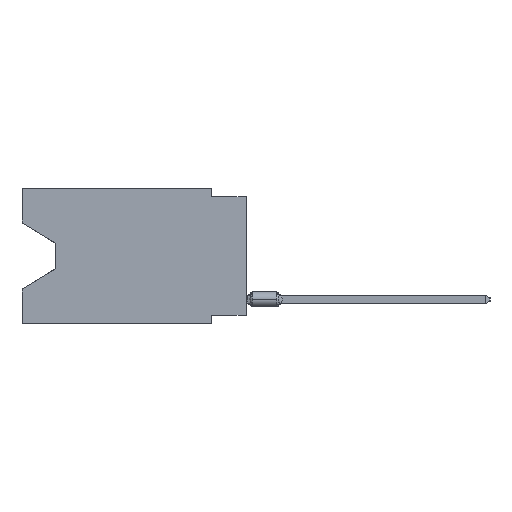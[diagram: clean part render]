
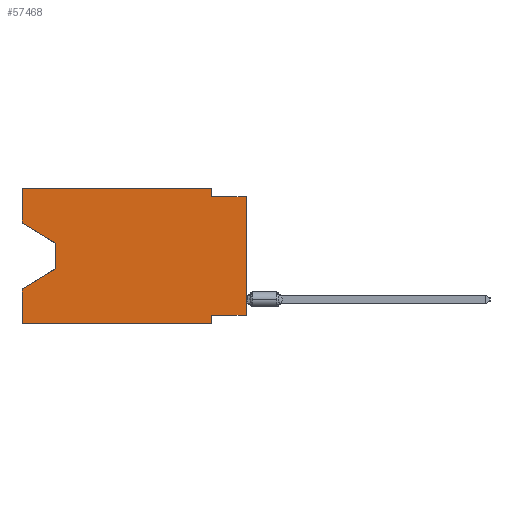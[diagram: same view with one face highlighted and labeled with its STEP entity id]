
A CAD part, left-side view. The second image highlights one B-rep face of the part: STEP entity #57468.
In plain terms, the highlighted planar face has unit normal (-1, 0, 0).
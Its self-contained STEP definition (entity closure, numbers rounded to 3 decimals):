
#312 = VERTEX_POINT ( 'NONE', #64722 ) ;
#390 = VERTEX_POINT ( 'NONE', #60776 ) ;
#616 = LINE ( 'NONE', #49810, #27023 ) ;
#1805 = VECTOR ( 'NONE', #11843, 1000. ) ;
#2131 = CARTESIAN_POINT ( 'NONE',  ( 0., 2.54, 0. ) ) ;
#2277 = DIRECTION ( 'NONE',  ( 0., 0., 1. ) ) ;
#3810 = VERTEX_POINT ( 'NONE', #54283 ) ;
#4911 = DIRECTION ( 'NONE',  ( 0., 0., -1. ) ) ;
#5344 = ORIENTED_EDGE ( 'NONE', *, *, #46273, .F. ) ;
#6207 = LINE ( 'NONE', #26187, #10376 ) ;
#6479 = EDGE_CURVE ( 'NONE', #29815, #59189, #6207, .T. ) ;
#7661 = VECTOR ( 'NONE', #58442, 1000. ) ;
#8578 = ORIENTED_EDGE ( 'NONE', *, *, #23154, .F. ) ;
#8912 = VERTEX_POINT ( 'NONE', #18530 ) ;
#9958 = VECTOR ( 'NONE', #48693, 1000. ) ;
#10316 = ORIENTED_EDGE ( 'NONE', *, *, #39422, .F. ) ;
#10376 = VECTOR ( 'NONE', #10479, 1000. ) ;
#10479 = DIRECTION ( 'NONE',  ( 0., 0., 1. ) ) ;
#11692 = CARTESIAN_POINT ( 'NONE',  ( 0., 16.383, 0. ) ) ;
#11843 = DIRECTION ( 'NONE',  ( 0., -1., 0. ) ) ;
#12703 = CARTESIAN_POINT ( 'NONE',  ( 0., 16.383, 0. ) ) ;
#13539 = ORIENTED_EDGE ( 'NONE', *, *, #14129, .T. ) ;
#14129 = EDGE_CURVE ( 'NONE', #24003, #54832, #16486, .T. ) ;
#15147 = VECTOR ( 'NONE', #36463, 1000. ) ;
#15238 = LINE ( 'NONE', #35218, #9958 ) ;
#15255 = CARTESIAN_POINT ( 'NONE',  ( 0., 0., -9.271 ) ) ;
#15559 = CARTESIAN_POINT ( 'NONE',  ( 0., 13.97, -4.013 ) ) ;
#15710 = EDGE_CURVE ( 'NONE', #23939, #8912, #48257, .T. ) ;
#16486 = LINE ( 'NONE', #56502, #15147 ) ;
#17256 = PLANE ( 'NONE',  #33274 ) ;
#17684 = CARTESIAN_POINT ( 'NONE',  ( 0., 0., -9.271 ) ) ;
#17859 = VECTOR ( 'NONE', #2277, 1000. ) ;
#18530 = CARTESIAN_POINT ( 'NONE',  ( 0., 2.54, -0.635 ) ) ;
#18812 = CARTESIAN_POINT ( 'NONE',  ( 0., 0., -0.635 ) ) ;
#19015 = EDGE_CURVE ( 'NONE', #54832, #312, #616, .T. ) ;
#21402 = VECTOR ( 'NONE', #40288, 1000. ) ;
#22529 = DIRECTION ( 'NONE',  ( 0., 0., 1. ) ) ;
#23154 = EDGE_CURVE ( 'NONE', #29815, #3810, #62627, .T. ) ;
#23583 = VERTEX_POINT ( 'NONE', #37598 ) ;
#23939 = VERTEX_POINT ( 'NONE', #2131 ) ;
#24003 = VERTEX_POINT ( 'NONE', #47031 ) ;
#26187 = CARTESIAN_POINT ( 'NONE',  ( 0., 0., 0. ) ) ;
#26450 = DIRECTION ( 'NONE',  ( 1., 0., 0. ) ) ;
#26814 = ORIENTED_EDGE ( 'NONE', *, *, #6479, .T. ) ;
#27023 = VECTOR ( 'NONE', #4911, 1000. ) ;
#27072 = VECTOR ( 'NONE', #22529, 1000. ) ;
#27795 = CARTESIAN_POINT ( 'NONE',  ( 0., 0., -0.635 ) ) ;
#28430 = ORIENTED_EDGE ( 'NONE', *, *, #40387, .F. ) ;
#28435 = DIRECTION ( 'NONE',  ( 0., -1., 0. ) ) ;
#29815 = VERTEX_POINT ( 'NONE', #15255 ) ;
#30987 = ORIENTED_EDGE ( 'NONE', *, *, #19015, .T. ) ;
#32422 = LINE ( 'NONE', #57045, #17859 ) ;
#33274 = AXIS2_PLACEMENT_3D ( 'NONE', #11692, #26450, #47416 ) ;
#33827 = CARTESIAN_POINT ( 'NONE',  ( 0., 2.54, 0. ) ) ;
#34056 = DIRECTION ( 'NONE',  ( 0., 1., 0. ) ) ;
#35218 = CARTESIAN_POINT ( 'NONE',  ( 0., 13.97, -5.893 ) ) ;
#35427 = ORIENTED_EDGE ( 'NONE', *, *, #64408, .T. ) ;
#36463 = DIRECTION ( 'NONE',  ( 0., -0.855, -0.519 ) ) ;
#37598 = CARTESIAN_POINT ( 'NONE',  ( 0., 16.383, -7.36 ) ) ;
#38418 = LINE ( 'NONE', #54181, #7661 ) ;
#39365 = EDGE_CURVE ( 'NONE', #312, #23583, #15238, .T. ) ;
#39422 = EDGE_CURVE ( 'NONE', #8912, #59189, #58309, .T. ) ;
#40288 = DIRECTION ( 'NONE',  ( 0., 0., -1. ) ) ;
#40387 = EDGE_CURVE ( 'NONE', #45921, #23939, #41336, .T. ) ;
#40996 = LINE ( 'NONE', #56087, #27072 ) ;
#41336 = LINE ( 'NONE', #12703, #61354 ) ;
#41977 = EDGE_CURVE ( 'NONE', #390, #23583, #40996, .T. ) ;
#41996 = CARTESIAN_POINT ( 'NONE',  ( 0., 16.383, 0. ) ) ;
#42727 = ORIENTED_EDGE ( 'NONE', *, *, #51479, .F. ) ;
#45921 = VERTEX_POINT ( 'NONE', #41996 ) ;
#46273 = EDGE_CURVE ( 'NONE', #24003, #45921, #32422, .T. ) ;
#47031 = CARTESIAN_POINT ( 'NONE',  ( 0., 16.383, -2.546 ) ) ;
#47416 = DIRECTION ( 'NONE',  ( 0., 0., -1. ) ) ;
#48257 = LINE ( 'NONE', #33827, #21402 ) ;
#48693 = DIRECTION ( 'NONE',  ( 0., 0.855, -0.519 ) ) ;
#49810 = CARTESIAN_POINT ( 'NONE',  ( 0., 13.97, -4.013 ) ) ;
#51479 = EDGE_CURVE ( 'NONE', #3810, #62570, #38418, .T. ) ;
#52166 = CARTESIAN_POINT ( 'NONE',  ( 0., 16.383, -9.906 ) ) ;
#53647 = VECTOR ( 'NONE', #34056, 1000. ) ;
#54181 = CARTESIAN_POINT ( 'NONE',  ( 0., 2.54, -9.906 ) ) ;
#54283 = CARTESIAN_POINT ( 'NONE',  ( 0., 2.54, -9.271 ) ) ;
#54832 = VERTEX_POINT ( 'NONE', #15559 ) ;
#55474 = EDGE_LOOP ( 'NONE', ( #13539, #30987, #63364, #58508, #35427, #42727, #8578, #26814, #10316, #62858, #28430, #5344 ) ) ;
#56087 = CARTESIAN_POINT ( 'NONE',  ( 0., 16.383, 0. ) ) ;
#56502 = CARTESIAN_POINT ( 'NONE',  ( 0., 16.383, -2.546 ) ) ;
#56771 = LINE ( 'NONE', #52166, #1805 ) ;
#57045 = CARTESIAN_POINT ( 'NONE',  ( 0., 16.383, 0. ) ) ;
#57468 = ADVANCED_FACE ( 'NONE', ( #57604 ), #17256, .F. ) ;
#57604 = FACE_OUTER_BOUND ( 'NONE', #55474, .T. ) ;
#57616 = CARTESIAN_POINT ( 'NONE',  ( 0., 2.54, -9.906 ) ) ;
#58298 = DIRECTION ( 'NONE',  ( 0., -1., 0. ) ) ;
#58309 = LINE ( 'NONE', #27795, #59198 ) ;
#58442 = DIRECTION ( 'NONE',  ( 0., 0., -1. ) ) ;
#58508 = ORIENTED_EDGE ( 'NONE', *, *, #41977, .F. ) ;
#59189 = VERTEX_POINT ( 'NONE', #18812 ) ;
#59198 = VECTOR ( 'NONE', #28435, 1000. ) ;
#60776 = CARTESIAN_POINT ( 'NONE',  ( 0., 16.383, -9.906 ) ) ;
#61354 = VECTOR ( 'NONE', #58298, 1000. ) ;
#62570 = VERTEX_POINT ( 'NONE', #57616 ) ;
#62627 = LINE ( 'NONE', #17684, #53647 ) ;
#62858 = ORIENTED_EDGE ( 'NONE', *, *, #15710, .F. ) ;
#63364 = ORIENTED_EDGE ( 'NONE', *, *, #39365, .T. ) ;
#64408 = EDGE_CURVE ( 'NONE', #390, #62570, #56771, .T. ) ;
#64722 = CARTESIAN_POINT ( 'NONE',  ( 0., 13.97, -5.893 ) ) ;
